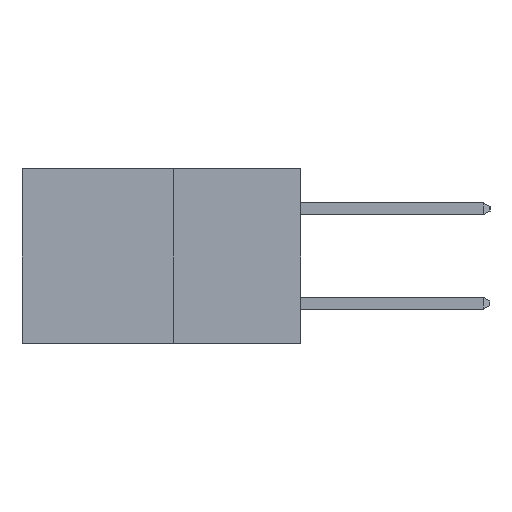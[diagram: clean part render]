
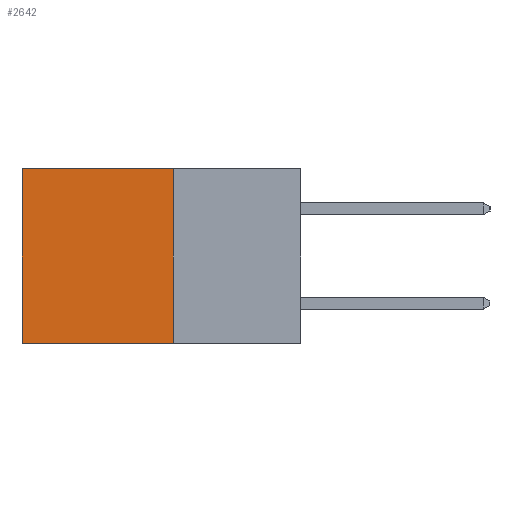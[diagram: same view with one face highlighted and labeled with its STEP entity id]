
A CAD part, left-side view. The second image highlights one B-rep face of the part: STEP entity #2642.
In plain terms, the highlighted planar face has unit normal (-1, 0, 0).
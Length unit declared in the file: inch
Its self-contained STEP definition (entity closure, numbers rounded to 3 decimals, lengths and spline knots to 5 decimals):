
#1110 = CARTESIAN_POINT ( 'NONE',  ( 0.277, 0.27, -0.37 ) ) ;
#2526 = VECTOR ( 'NONE', #12140, 39.37008 ) ;
#2642 = ADVANCED_FACE ( 'NONE', ( #14236 ), #19491, .F. ) ;
#3427 = EDGE_CURVE ( 'NONE', #6825, #15883, #19112, .T. ) ;
#3620 = CARTESIAN_POINT ( 'NONE',  ( 0.277, 0.27, -0.37 ) ) ;
#4501 = VERTEX_POINT ( 'NONE', #23831 ) ;
#5445 = VECTOR ( 'NONE', #17843, 39.37008 ) ;
#6268 = EDGE_CURVE ( 'NONE', #4501, #15883, #25920, .T. ) ;
#6611 = ORIENTED_EDGE ( 'NONE', *, *, #3427, .F. ) ;
#6825 = VERTEX_POINT ( 'NONE', #3620 ) ;
#8967 = CARTESIAN_POINT ( 'NONE',  ( 0.277, 0.59, -0.37 ) ) ;
#10090 = CARTESIAN_POINT ( 'NONE',  ( 0.277, 0.27, 0. ) ) ;
#10965 = ORIENTED_EDGE ( 'NONE', *, *, #22914, .F. ) ;
#11414 = LINE ( 'NONE', #15574, #5445 ) ;
#11544 = CARTESIAN_POINT ( 'NONE',  ( 0.277, 0.59, -0.37 ) ) ;
#11766 = DIRECTION ( 'NONE',  ( 0., 0., -1. ) ) ;
#11778 = AXIS2_PLACEMENT_3D ( 'NONE', #1110, #25803, #26647 ) ;
#12140 = DIRECTION ( 'NONE',  ( 0., 1., 0. ) ) ;
#14236 = FACE_OUTER_BOUND ( 'NONE', #28901, .T. ) ;
#14487 = LINE ( 'NONE', #27770, #2526 ) ;
#14725 = VECTOR ( 'NONE', #11766, 39.37008 ) ;
#15574 = CARTESIAN_POINT ( 'NONE',  ( 0.277, 0.27, -0.37 ) ) ;
#15883 = VERTEX_POINT ( 'NONE', #8967 ) ;
#17165 = VERTEX_POINT ( 'NONE', #10090 ) ;
#17843 = DIRECTION ( 'NONE',  ( 0., 0., -1. ) ) ;
#18425 = ORIENTED_EDGE ( 'NONE', *, *, #24334, .T. ) ;
#19112 = LINE ( 'NONE', #26287, #23656 ) ;
#19491 = PLANE ( 'NONE',  #11778 ) ;
#22914 = EDGE_CURVE ( 'NONE', #17165, #6825, #11414, .T. ) ;
#23151 = ORIENTED_EDGE ( 'NONE', *, *, #6268, .T. ) ;
#23656 = VECTOR ( 'NONE', #26060, 39.37008 ) ;
#23831 = CARTESIAN_POINT ( 'NONE',  ( 0.277, 0.59, 0. ) ) ;
#24334 = EDGE_CURVE ( 'NONE', #17165, #4501, #14487, .T. ) ;
#25803 = DIRECTION ( 'NONE',  ( 1., 0., 0. ) ) ;
#25920 = LINE ( 'NONE', #11544, #14725 ) ;
#26060 = DIRECTION ( 'NONE',  ( 0., 1., 0. ) ) ;
#26287 = CARTESIAN_POINT ( 'NONE',  ( 0.277, 0.27, -0.37 ) ) ;
#26647 = DIRECTION ( 'NONE',  ( 0., 0., -1. ) ) ;
#27770 = CARTESIAN_POINT ( 'NONE',  ( 0.277, 0.27, 0. ) ) ;
#28901 = EDGE_LOOP ( 'NONE', ( #23151, #6611, #10965, #18425 ) ) ;
